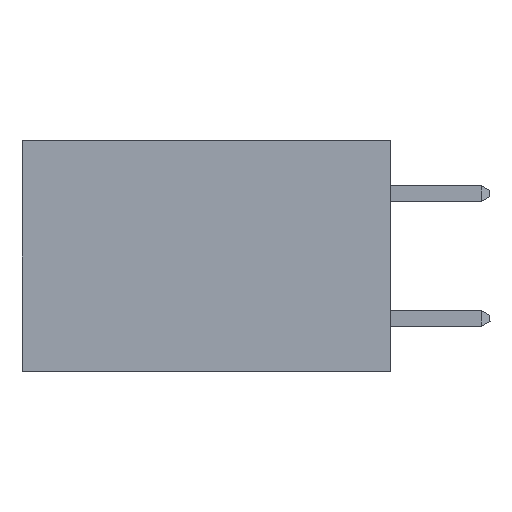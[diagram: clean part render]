
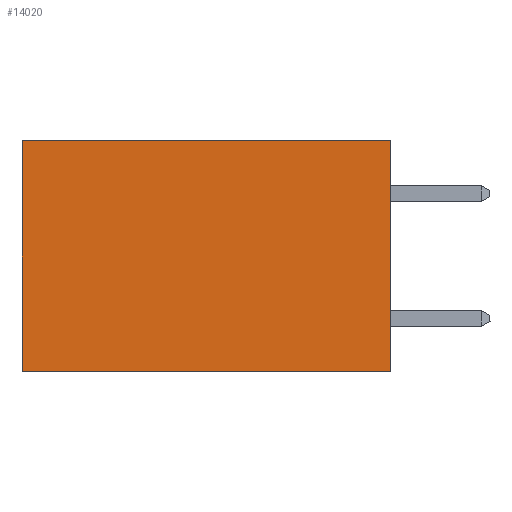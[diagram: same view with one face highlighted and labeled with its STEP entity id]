
A CAD part, left-side view. The second image highlights one B-rep face of the part: STEP entity #14020.
In plain terms, the highlighted planar face has unit normal (-1, 0, 0).
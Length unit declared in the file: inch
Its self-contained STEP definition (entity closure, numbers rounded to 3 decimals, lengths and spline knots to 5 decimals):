
#424 = DIRECTION ( 'NONE',  ( 0., 0., -1. ) ) ;
#457 = VECTOR ( 'NONE', #424, 39.37008 ) ;
#1514 = VERTEX_POINT ( 'NONE', #15136 ) ;
#1601 = CARTESIAN_POINT ( 'NONE',  ( 0.277, 0., -0.37 ) ) ;
#2149 = CARTESIAN_POINT ( 'NONE',  ( 0.277, 0.59, 0. ) ) ;
#2281 = VECTOR ( 'NONE', #12471, 39.37008 ) ;
#3590 = DIRECTION ( 'NONE',  ( 1., 0., 0. ) ) ;
#3835 = ORIENTED_EDGE ( 'NONE', *, *, #22581, .F. ) ;
#4021 = AXIS2_PLACEMENT_3D ( 'NONE', #1601, #3590, #17113 ) ;
#4164 = ORIENTED_EDGE ( 'NONE', *, *, #4733, .T. ) ;
#4733 = EDGE_CURVE ( 'NONE', #17858, #12152, #22883, .T. ) ;
#4804 = ORIENTED_EDGE ( 'NONE', *, *, #14105, .T. ) ;
#5669 = VECTOR ( 'NONE', #7680, 39.37008 ) ;
#7680 = DIRECTION ( 'NONE',  ( 0., 0., -1. ) ) ;
#9020 = CARTESIAN_POINT ( 'NONE',  ( 0.277, 0.59, -0.37 ) ) ;
#9705 = DIRECTION ( 'NONE',  ( 0., 1., 0. ) ) ;
#9946 = LINE ( 'NONE', #23249, #14480 ) ;
#10211 = LINE ( 'NONE', #23124, #5669 ) ;
#12047 = FACE_OUTER_BOUND ( 'NONE', #18947, .T. ) ;
#12152 = VERTEX_POINT ( 'NONE', #2149 ) ;
#12388 = CARTESIAN_POINT ( 'NONE',  ( 0.277, 0., 0. ) ) ;
#12426 = VERTEX_POINT ( 'NONE', #9020 ) ;
#12471 = DIRECTION ( 'NONE',  ( 0., 1., 0. ) ) ;
#13434 = EDGE_CURVE ( 'NONE', #1514, #12426, #9946, .T. ) ;
#14020 = ADVANCED_FACE ( 'NONE', ( #12047 ), #24816, .F. ) ;
#14105 = EDGE_CURVE ( 'NONE', #12152, #12426, #10211, .T. ) ;
#14480 = VECTOR ( 'NONE', #9705, 39.37008 ) ;
#15136 = CARTESIAN_POINT ( 'NONE',  ( 0.277, 0., -0.37 ) ) ;
#15959 = LINE ( 'NONE', #23668, #457 ) ;
#16433 = CARTESIAN_POINT ( 'NONE',  ( 0.277, 0., 0. ) ) ;
#17113 = DIRECTION ( 'NONE',  ( 0., 0., -1. ) ) ;
#17858 = VERTEX_POINT ( 'NONE', #16433 ) ;
#18947 = EDGE_LOOP ( 'NONE', ( #4804, #24150, #3835, #4164 ) ) ;
#22581 = EDGE_CURVE ( 'NONE', #17858, #1514, #15959, .T. ) ;
#22883 = LINE ( 'NONE', #12388, #2281 ) ;
#23124 = CARTESIAN_POINT ( 'NONE',  ( 0.277, 0.59, -0.37 ) ) ;
#23249 = CARTESIAN_POINT ( 'NONE',  ( 0.277, 0., -0.37 ) ) ;
#23668 = CARTESIAN_POINT ( 'NONE',  ( 0.277, 0., -0.37 ) ) ;
#24150 = ORIENTED_EDGE ( 'NONE', *, *, #13434, .F. ) ;
#24816 = PLANE ( 'NONE',  #4021 ) ;
